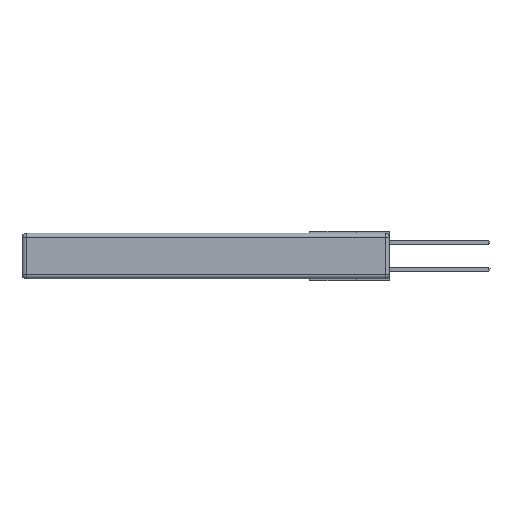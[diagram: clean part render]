
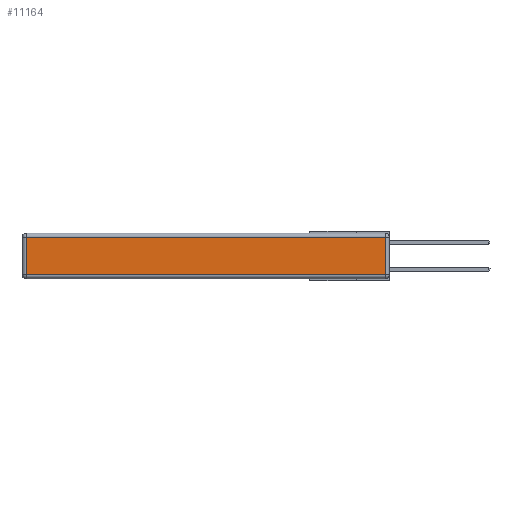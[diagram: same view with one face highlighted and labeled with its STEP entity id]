
A CAD part, left-side view. The second image highlights one B-rep face of the part: STEP entity #11164.
In plain terms, the highlighted planar face has unit normal (-1, 0, 0).
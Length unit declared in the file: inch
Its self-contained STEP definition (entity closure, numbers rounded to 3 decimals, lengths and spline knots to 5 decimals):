
#64 = ORIENTED_EDGE ( 'NONE', *, *, #11432, .T. ) ;
#420 = ORIENTED_EDGE ( 'NONE', *, *, #11005, .T. ) ;
#519 = LINE ( 'NONE', #13317, #11245 ) ;
#631 = ORIENTED_EDGE ( 'NONE', *, *, #1305, .T. ) ;
#1305 = EDGE_CURVE ( 'NONE', #5382, #8331, #6718, .T. ) ;
#1904 = ORIENTED_EDGE ( 'NONE', *, *, #4468, .T. ) ;
#2052 = CARTESIAN_POINT ( 'NONE',  ( 0., 0., -0.343 ) ) ;
#2523 = VECTOR ( 'NONE', #9598, 39.37008 ) ;
#2606 = DIRECTION ( 'NONE',  ( 0., -1., 0. ) ) ;
#3106 = CARTESIAN_POINT ( 'NONE',  ( 0., 0.03, -0.343 ) ) ;
#4262 = VECTOR ( 'NONE', #2606, 39.37008 ) ;
#4468 = EDGE_CURVE ( 'NONE', #8360, #6570, #5949, .T. ) ;
#5382 = VERTEX_POINT ( 'NONE', #10681 ) ;
#5617 = DIRECTION ( 'NONE',  ( 0., 1., 0. ) ) ;
#5949 = LINE ( 'NONE', #8536, #13149 ) ;
#6330 = AXIS2_PLACEMENT_3D ( 'NONE', #2052, #10955, #13686 ) ;
#6570 = VERTEX_POINT ( 'NONE', #10306 ) ;
#6718 = LINE ( 'NONE', #3106, #2523 ) ;
#7232 = PLANE ( 'NONE',  #6330 ) ;
#8249 = FACE_OUTER_BOUND ( 'NONE', #11158, .T. ) ;
#8331 = VERTEX_POINT ( 'NONE', #12495 ) ;
#8360 = VERTEX_POINT ( 'NONE', #14945 ) ;
#8536 = CARTESIAN_POINT ( 'NONE',  ( 0., 2.72, -0.343 ) ) ;
#9598 = DIRECTION ( 'NONE',  ( 0., 0., 1. ) ) ;
#10306 = CARTESIAN_POINT ( 'NONE',  ( 0., 2.72, -0.313 ) ) ;
#10681 = CARTESIAN_POINT ( 'NONE',  ( 0., 0.03, -0.313 ) ) ;
#10955 = DIRECTION ( 'NONE',  ( -1., 0., 0. ) ) ;
#11005 = EDGE_CURVE ( 'NONE', #8331, #8360, #519, .T. ) ;
#11158 = EDGE_LOOP ( 'NONE', ( #64, #631, #420, #1904 ) ) ;
#11164 = ADVANCED_FACE ( 'NONE', ( #8249 ), #7232, .T. ) ;
#11245 = VECTOR ( 'NONE', #5617, 39.37008 ) ;
#11432 = EDGE_CURVE ( 'NONE', #6570, #5382, #15802, .T. ) ;
#11632 = CARTESIAN_POINT ( 'NONE',  ( 0., 0., -0.313 ) ) ;
#12329 = DIRECTION ( 'NONE',  ( 0., 0., -1. ) ) ;
#12495 = CARTESIAN_POINT ( 'NONE',  ( 0., 0.03, -0.03 ) ) ;
#13149 = VECTOR ( 'NONE', #12329, 39.37008 ) ;
#13317 = CARTESIAN_POINT ( 'NONE',  ( 0., 2.75, -0.03 ) ) ;
#13686 = DIRECTION ( 'NONE',  ( 0., 0., 1. ) ) ;
#14945 = CARTESIAN_POINT ( 'NONE',  ( 0., 2.72, -0.03 ) ) ;
#15802 = LINE ( 'NONE', #11632, #4262 ) ;
